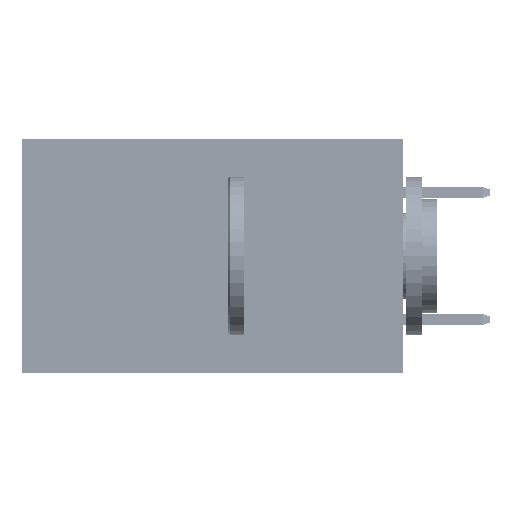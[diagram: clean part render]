
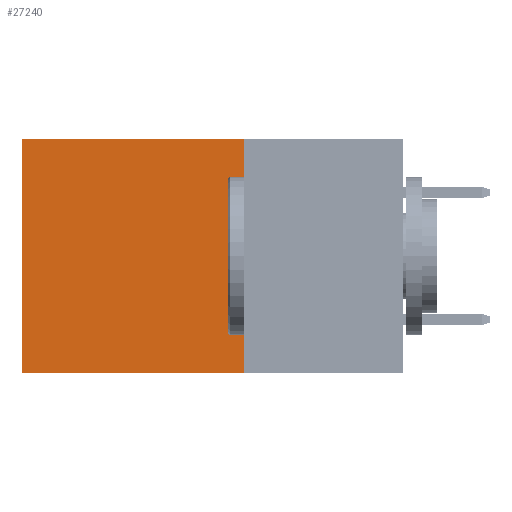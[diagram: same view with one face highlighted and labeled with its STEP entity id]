
A CAD part, left-side view. The second image highlights one B-rep face of the part: STEP entity #27240.
In plain terms, the highlighted planar face has unit normal (-1, 0, 0).
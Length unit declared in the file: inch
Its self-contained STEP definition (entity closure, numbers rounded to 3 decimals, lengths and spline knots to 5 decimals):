
#585 = EDGE_LOOP ( 'NONE', ( #28826, #33504, #31980, #16499 ) ) ;
#2975 = AXIS2_PLACEMENT_3D ( 'NONE', #26838, #7166, #10040 ) ;
#6163 = CARTESIAN_POINT ( 'NONE',  ( 0.2875, 0.6, 0. ) ) ;
#7166 = DIRECTION ( 'NONE',  ( 1., 0., 0. ) ) ;
#8785 = LINE ( 'NONE', #24782, #17307 ) ;
#10040 = DIRECTION ( 'NONE',  ( 0., 0., -1. ) ) ;
#11491 = LINE ( 'NONE', #11742, #37229 ) ;
#11742 = CARTESIAN_POINT ( 'NONE',  ( 0.2875, 0.25, 0. ) ) ;
#13595 = CARTESIAN_POINT ( 'NONE',  ( 0.2875, 0.25, 0. ) ) ;
#13695 = EDGE_CURVE ( 'NONE', #37459, #36380, #37954, .T. ) ;
#14175 = CARTESIAN_POINT ( 'NONE',  ( 0.2875, 0.6, 0. ) ) ;
#16499 = ORIENTED_EDGE ( 'NONE', *, *, #18878, .T. ) ;
#17006 = CARTESIAN_POINT ( 'NONE',  ( 0.2875, 0.25, -0.37 ) ) ;
#17307 = VECTOR ( 'NONE', #32437, 39.37008 ) ;
#17937 = DIRECTION ( 'NONE',  ( 0., 0., -1. ) ) ;
#18145 = PLANE ( 'NONE',  #2975 ) ;
#18878 = EDGE_CURVE ( 'NONE', #43719, #37459, #11491, .T. ) ;
#21393 = DIRECTION ( 'NONE',  ( 0., 0., -1. ) ) ;
#22161 = LINE ( 'NONE', #29271, #22801 ) ;
#22801 = VECTOR ( 'NONE', #21393, 39.37008 ) ;
#23875 = DIRECTION ( 'NONE',  ( 0., 1., 0. ) ) ;
#24782 = CARTESIAN_POINT ( 'NONE',  ( 0.2875, 0.25, -0.37 ) ) ;
#26838 = CARTESIAN_POINT ( 'NONE',  ( 0.2875, 0.25, 0. ) ) ;
#27240 = ADVANCED_FACE ( 'NONE', ( #38678 ), #18145, .F. ) ;
#27579 = VECTOR ( 'NONE', #17937, 39.37008 ) ;
#28826 = ORIENTED_EDGE ( 'NONE', *, *, #13695, .T. ) ;
#29271 = CARTESIAN_POINT ( 'NONE',  ( 0.2875, 0.25, 0. ) ) ;
#31980 = ORIENTED_EDGE ( 'NONE', *, *, #41520, .F. ) ;
#32437 = DIRECTION ( 'NONE',  ( 0., 1., 0. ) ) ;
#33504 = ORIENTED_EDGE ( 'NONE', *, *, #34117, .F. ) ;
#33573 = CARTESIAN_POINT ( 'NONE',  ( 0.2875, 0.6, -0.37 ) ) ;
#34117 = EDGE_CURVE ( 'NONE', #40951, #36380, #8785, .T. ) ;
#36380 = VERTEX_POINT ( 'NONE', #33573 ) ;
#37229 = VECTOR ( 'NONE', #23875, 39.37008 ) ;
#37459 = VERTEX_POINT ( 'NONE', #14175 ) ;
#37954 = LINE ( 'NONE', #6163, #27579 ) ;
#38678 = FACE_OUTER_BOUND ( 'NONE', #585, .T. ) ;
#40951 = VERTEX_POINT ( 'NONE', #17006 ) ;
#41520 = EDGE_CURVE ( 'NONE', #43719, #40951, #22161, .T. ) ;
#43719 = VERTEX_POINT ( 'NONE', #13595 ) ;
